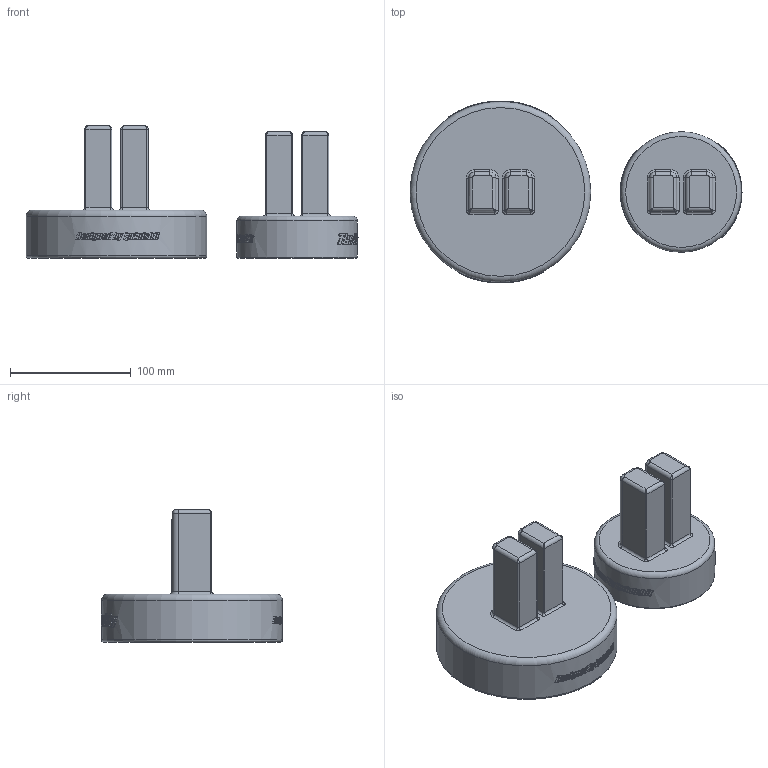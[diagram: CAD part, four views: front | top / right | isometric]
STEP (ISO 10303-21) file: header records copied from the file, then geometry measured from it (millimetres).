
FILE_DESCRIPTION(/* description */ (''),/* implementation_level */ '2;1');
FILE_NAME(/* name */ 'Glocknofsky Stand v4.step',/* time_stamp */ '2022-03-26T10:54:02-04:00',/* author */ (''),/* organization */ (''),/* preprocessor_version */ 'ST-DEVELOPER v18.1',/* originating_system */ 'Autodesk Translation Framework v10.13.0.1454',/* authorisation */ '');
FILE_SCHEMA (('AUTOMOTIVE_DESIGN { 1 0 10303 214 3 1 1 }'));
Products named in the file (2): Glocknofsky Stand; Component1
Assembly tree (1 placements, depth 2):
  Glocknofsky Stand
    Component1
Bounding box: 275.5 x 151 x 110 mm (x, y, z)
Volume: 1183817.6 mm3; surface area: 108617.7 mm2
Topology: 2 solids, 2 shells, 1598 faces, 4420 edges, 2916 vertices
Faces by surface type: bspline 852, plane 580, cylinder 146, torus 20
Full cylindrical faces by diameter (mm): 100 x1, 150 x1
Entity records: 94105 total; most frequent: CARTESIAN_POINT 57948, ORIENTED_EDGE 8824, DIRECTION 5476, EDGE_CURVE 4412, VERTEX_POINT 2916, AXIS2_PLACEMENT_3D 1991, EDGE_LOOP 1696, B_SPLINE_CURVE_WITH_KNOTS 1674
